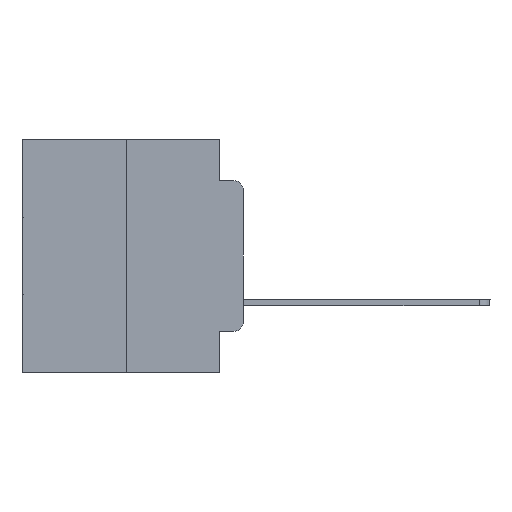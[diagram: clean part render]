
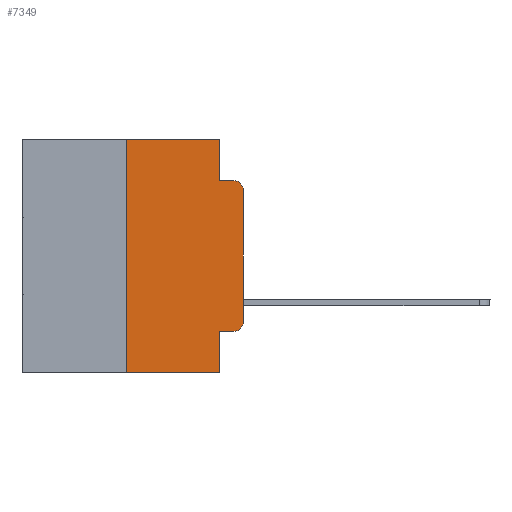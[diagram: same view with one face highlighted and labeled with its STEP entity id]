
A CAD part, left-side view. The second image highlights one B-rep face of the part: STEP entity #7349.
In plain terms, the highlighted planar face has unit normal (-1, 0, 0).
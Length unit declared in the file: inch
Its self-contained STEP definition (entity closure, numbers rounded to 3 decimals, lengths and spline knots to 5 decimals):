
#12 = CARTESIAN_POINT ( 'NONE',  ( 0., 0.473, -0.5 ) ) ;
#183 = ORIENTED_EDGE ( 'NONE', *, *, #13348, .F. ) ;
#376 = AXIS2_PLACEMENT_3D ( 'NONE', #23885, #14746, #23070 ) ;
#991 = EDGE_CURVE ( 'NONE', #6341, #3755, #18085, .T. ) ;
#1096 = VECTOR ( 'NONE', #9887, 39.37008 ) ;
#1785 = DIRECTION ( 'NONE',  ( 0., 0., 1. ) ) ;
#1820 = LINE ( 'NONE', #10013, #26751 ) ;
#1947 = VERTEX_POINT ( 'NONE', #4205 ) ;
#2023 = VECTOR ( 'NONE', #6679, 39.37008 ) ;
#2300 = DIRECTION ( 'NONE',  ( 0., -1., 0. ) ) ;
#2381 = ORIENTED_EDGE ( 'NONE', *, *, #22301, .T. ) ;
#3137 = LINE ( 'NONE', #5667, #16511 ) ;
#3755 = VERTEX_POINT ( 'NONE', #11139 ) ;
#4205 = CARTESIAN_POINT ( 'NONE',  ( 0., 0.02, -0.4115 ) ) ;
#4478 = VECTOR ( 'NONE', #16142, 39.37008 ) ;
#4491 = ORIENTED_EDGE ( 'NONE', *, *, #23893, .F. ) ;
#4525 = LINE ( 'NONE', #13113, #1096 ) ;
#4793 = EDGE_CURVE ( 'NONE', #8113, #1947, #22907, .T. ) ;
#5080 = ORIENTED_EDGE ( 'NONE', *, *, #24449, .F. ) ;
#5667 = CARTESIAN_POINT ( 'NONE',  ( 0., 0.051, 0. ) ) ;
#5870 = EDGE_LOOP ( 'NONE', ( #25110, #11707, #4491, #11052, #183, #19467, #8409, #5080, #22642, #2381 ) ) ;
#5931 = AXIS2_PLACEMENT_3D ( 'NONE', #26903, #26619, #11674 ) ;
#6076 = CARTESIAN_POINT ( 'NONE',  ( 0., 0.051, -0.0885 ) ) ;
#6341 = VERTEX_POINT ( 'NONE', #22048 ) ;
#6679 = DIRECTION ( 'NONE',  ( 0., 0., 1. ) ) ;
#6732 = CARTESIAN_POINT ( 'NONE',  ( 0., 0.051, -0.5 ) ) ;
#6742 = CARTESIAN_POINT ( 'NONE',  ( 0., 0.051, -0.0885 ) ) ;
#6913 = DIRECTION ( 'NONE',  ( -1., 0., 0. ) ) ;
#7309 = PLANE ( 'NONE',  #376 ) ;
#7349 = ADVANCED_FACE ( 'NONE', ( #15894 ), #7309, .F. ) ;
#8113 = VERTEX_POINT ( 'NONE', #21586 ) ;
#8149 = CARTESIAN_POINT ( 'NONE',  ( 0., 0., 0. ) ) ;
#8409 = ORIENTED_EDGE ( 'NONE', *, *, #17791, .T. ) ;
#8825 = VERTEX_POINT ( 'NONE', #20539 ) ;
#9115 = DIRECTION ( 'NONE',  ( 0., -1., 0. ) ) ;
#9887 = DIRECTION ( 'NONE',  ( 0., -1., 0. ) ) ;
#10013 = CARTESIAN_POINT ( 'NONE',  ( 0., 0.051, 0. ) ) ;
#10018 = DIRECTION ( 'NONE',  ( 0., 0., -1. ) ) ;
#11052 = ORIENTED_EDGE ( 'NONE', *, *, #27503, .F. ) ;
#11139 = CARTESIAN_POINT ( 'NONE',  ( 0., 0.02, -0.0885 ) ) ;
#11674 = DIRECTION ( 'NONE',  ( 0., 0., -1. ) ) ;
#11707 = ORIENTED_EDGE ( 'NONE', *, *, #991, .T. ) ;
#12298 = AXIS2_PLACEMENT_3D ( 'NONE', #25942, #6913, #21858 ) ;
#12674 = VERTEX_POINT ( 'NONE', #19373 ) ;
#12832 = VERTEX_POINT ( 'NONE', #22479 ) ;
#13113 = CARTESIAN_POINT ( 'NONE',  ( 0., 0.473, 0. ) ) ;
#13348 = EDGE_CURVE ( 'NONE', #8825, #12832, #4525, .T. ) ;
#13602 = LINE ( 'NONE', #6742, #21318 ) ;
#13716 = VECTOR ( 'NONE', #1785, 39.37008 ) ;
#14164 = VERTEX_POINT ( 'NONE', #6732 ) ;
#14746 = DIRECTION ( 'NONE',  ( 1., 0., 0. ) ) ;
#15052 = EDGE_CURVE ( 'NONE', #12674, #6341, #21128, .T. ) ;
#15894 = FACE_OUTER_BOUND ( 'NONE', #5870, .T. ) ;
#16142 = DIRECTION ( 'NONE',  ( 0., -1., 0. ) ) ;
#16511 = VECTOR ( 'NONE', #10018, 39.37008 ) ;
#16557 = CARTESIAN_POINT ( 'NONE',  ( 0., 0.051, -0.4115 ) ) ;
#17791 = EDGE_CURVE ( 'NONE', #21457, #14164, #23739, .T. ) ;
#18085 = CIRCLE ( 'NONE', #5931, 0.02 ) ;
#18176 = CARTESIAN_POINT ( 'NONE',  ( 0., 0.25, 0. ) ) ;
#18344 = DIRECTION ( 'NONE',  ( 0., 0., -1. ) ) ;
#19061 = CIRCLE ( 'NONE', #12298, 0.02 ) ;
#19373 = CARTESIAN_POINT ( 'NONE',  ( 0., 0., -0.3915 ) ) ;
#19467 = ORIENTED_EDGE ( 'NONE', *, *, #26056, .F. ) ;
#20539 = CARTESIAN_POINT ( 'NONE',  ( 0., 0.25, 0. ) ) ;
#21128 = LINE ( 'NONE', #8149, #13716 ) ;
#21318 = VECTOR ( 'NONE', #9115, 39.37008 ) ;
#21457 = VERTEX_POINT ( 'NONE', #23921 ) ;
#21586 = CARTESIAN_POINT ( 'NONE',  ( 0., 0.051, -0.4115 ) ) ;
#21858 = DIRECTION ( 'NONE',  ( 0., 0., -1. ) ) ;
#22048 = CARTESIAN_POINT ( 'NONE',  ( 0., 0., -0.1085 ) ) ;
#22246 = VERTEX_POINT ( 'NONE', #6076 ) ;
#22279 = LINE ( 'NONE', #18176, #2023 ) ;
#22301 = EDGE_CURVE ( 'NONE', #1947, #12674, #19061, .T. ) ;
#22479 = CARTESIAN_POINT ( 'NONE',  ( 0., 0.051, 0. ) ) ;
#22642 = ORIENTED_EDGE ( 'NONE', *, *, #4793, .T. ) ;
#22907 = LINE ( 'NONE', #16557, #4478 ) ;
#23070 = DIRECTION ( 'NONE',  ( 0., 0., -1. ) ) ;
#23307 = VECTOR ( 'NONE', #2300, 39.37008 ) ;
#23739 = LINE ( 'NONE', #12, #23307 ) ;
#23885 = CARTESIAN_POINT ( 'NONE',  ( 0., 0.473, 0. ) ) ;
#23893 = EDGE_CURVE ( 'NONE', #22246, #3755, #13602, .T. ) ;
#23921 = CARTESIAN_POINT ( 'NONE',  ( 0., 0.25, -0.5 ) ) ;
#24449 = EDGE_CURVE ( 'NONE', #8113, #14164, #1820, .T. ) ;
#25110 = ORIENTED_EDGE ( 'NONE', *, *, #15052, .T. ) ;
#25942 = CARTESIAN_POINT ( 'NONE',  ( 0., 0.02, -0.3915 ) ) ;
#26056 = EDGE_CURVE ( 'NONE', #21457, #8825, #22279, .T. ) ;
#26619 = DIRECTION ( 'NONE',  ( -1., 0., 0. ) ) ;
#26751 = VECTOR ( 'NONE', #18344, 39.37008 ) ;
#26903 = CARTESIAN_POINT ( 'NONE',  ( 0., 0.02, -0.1085 ) ) ;
#27503 = EDGE_CURVE ( 'NONE', #12832, #22246, #3137, .T. ) ;
